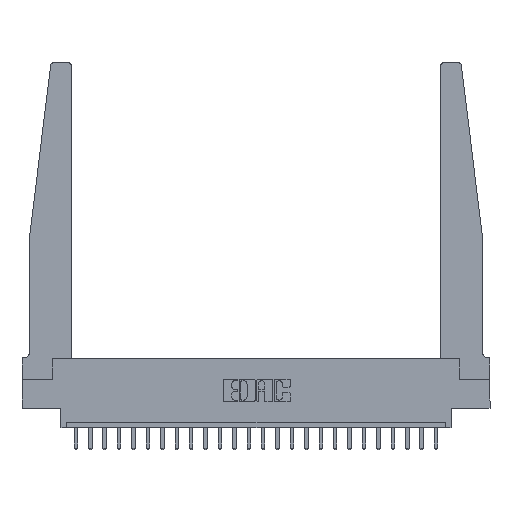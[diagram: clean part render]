
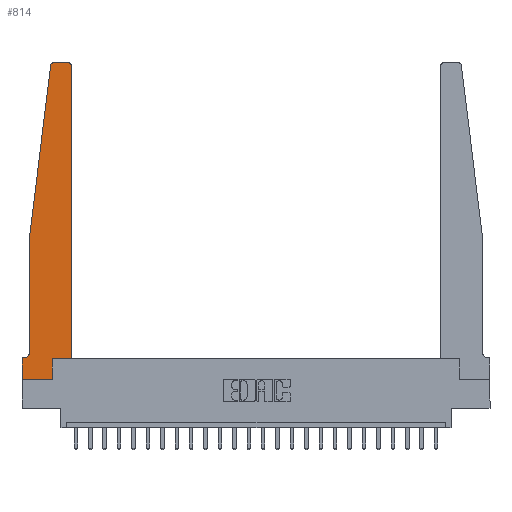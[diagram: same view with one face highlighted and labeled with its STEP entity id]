
A CAD part, top view. The second image highlights one B-rep face of the part: STEP entity #814.
In plain terms, the highlighted planar face has unit normal (0, 0, 1).
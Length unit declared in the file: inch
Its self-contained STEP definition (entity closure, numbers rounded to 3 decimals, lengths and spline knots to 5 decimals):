
#510 = CARTESIAN_POINT ( 'NONE',  ( 0.015, 0.1875, 0.37 ) ) ;
#647 = LINE ( 'NONE', #21854, #4325 ) ;
#814 = ADVANCED_FACE ( 'NONE', ( #14482 ), #22497, .T. ) ;
#943 = VECTOR ( 'NONE', #6972, 39.37008 ) ;
#951 = CARTESIAN_POINT ( 'NONE',  ( 0., 0.1875, 0.37 ) ) ;
#1083 = DIRECTION ( 'NONE',  ( -0.122, -0.992, 0. ) ) ;
#1521 = CARTESIAN_POINT ( 'NONE',  ( 0.065, 0.1875, 0.37 ) ) ;
#2001 = EDGE_CURVE ( 'NONE', #9670, #10453, #11016, .T. ) ;
#2574 = ORIENTED_EDGE ( 'NONE', *, *, #3898, .T. ) ;
#2710 = VECTOR ( 'NONE', #20723, 39.37008 ) ;
#2790 = ORIENTED_EDGE ( 'NONE', *, *, #19519, .T. ) ;
#3064 = ORIENTED_EDGE ( 'NONE', *, *, #8582, .T. ) ;
#3898 = EDGE_CURVE ( 'NONE', #12714, #7843, #4428, .T. ) ;
#3945 = CARTESIAN_POINT ( 'NONE',  ( 0.395, 2.72, 0.37 ) ) ;
#4252 = CARTESIAN_POINT ( 'NONE',  ( 0.395, 2.75, 0.37 ) ) ;
#4325 = VECTOR ( 'NONE', #9304, 39.37008 ) ;
#4428 = LINE ( 'NONE', #17457, #2710 ) ;
#4794 = CARTESIAN_POINT ( 'NONE',  ( 0.425, 0.18, 0.37 ) ) ;
#5068 = DIRECTION ( 'NONE',  ( -1., 0., 0. ) ) ;
#5776 = DIRECTION ( 'NONE',  ( 0., 0., 1. ) ) ;
#5869 = EDGE_LOOP ( 'NONE', ( #23331, #13779, #8024, #22298, #11572, #3064, #17739, #11945, #2790, #2574, #11406, #8471 ) ) ;
#5877 = LINE ( 'NONE', #12318, #21608 ) ;
#6385 = CARTESIAN_POINT ( 'NONE',  ( 0.425, 2.72, 0.37 ) ) ;
#6489 = DIRECTION ( 'NONE',  ( 1., 0., 0. ) ) ;
#6539 = DIRECTION ( 'NONE',  ( -1., 0., 0. ) ) ;
#6719 = CARTESIAN_POINT ( 'NONE',  ( 0.2605, 0.18, 0.37 ) ) ;
#6972 = DIRECTION ( 'NONE',  ( -1., 0., 0. ) ) ;
#7675 = VERTEX_POINT ( 'NONE', #22727 ) ;
#7843 = VERTEX_POINT ( 'NONE', #10070 ) ;
#8024 = ORIENTED_EDGE ( 'NONE', *, *, #13132, .T. ) ;
#8038 = LINE ( 'NONE', #4794, #15122 ) ;
#8423 = EDGE_CURVE ( 'NONE', #10469, #11655, #21215, .T. ) ;
#8471 = ORIENTED_EDGE ( 'NONE', *, *, #2001, .T. ) ;
#8582 = EDGE_CURVE ( 'NONE', #20095, #7675, #20371, .T. ) ;
#9175 = EDGE_CURVE ( 'NONE', #10453, #10469, #10291, .T. ) ;
#9304 = DIRECTION ( 'NONE',  ( 0., -1., 0. ) ) ;
#9467 = AXIS2_PLACEMENT_3D ( 'NONE', #951, #15490, #6489 ) ;
#9670 = VERTEX_POINT ( 'NONE', #6385 ) ;
#10070 = CARTESIAN_POINT ( 'NONE',  ( 0.425, 0.18, 0.37 ) ) ;
#10280 = DIRECTION ( 'NONE',  ( 0., 1., 0. ) ) ;
#10291 = LINE ( 'NONE', #16037, #12256 ) ;
#10453 = VERTEX_POINT ( 'NONE', #4252 ) ;
#10469 = VERTEX_POINT ( 'NONE', #20608 ) ;
#10473 = CARTESIAN_POINT ( 'NONE',  ( 0.065, 1.25, 0.37 ) ) ;
#10687 = DIRECTION ( 'NONE',  ( 1., 0., 0. ) ) ;
#11016 = CIRCLE ( 'NONE', #13734, 0.03 ) ;
#11231 = VECTOR ( 'NONE', #12220, 39.37008 ) ;
#11406 = ORIENTED_EDGE ( 'NONE', *, *, #15987, .T. ) ;
#11572 = ORIENTED_EDGE ( 'NONE', *, *, #11796, .T. ) ;
#11655 = VERTEX_POINT ( 'NONE', #13926 ) ;
#11796 = EDGE_CURVE ( 'NONE', #17698, #20095, #22821, .T. ) ;
#11915 = CARTESIAN_POINT ( 'NONE',  ( 0.015, 0.2375, 0.37 ) ) ;
#11945 = ORIENTED_EDGE ( 'NONE', *, *, #14440, .T. ) ;
#12220 = DIRECTION ( 'NONE',  ( 0., -1., 0. ) ) ;
#12256 = VECTOR ( 'NONE', #5068, 39.37008 ) ;
#12270 = VERTEX_POINT ( 'NONE', #10473 ) ;
#12318 = CARTESIAN_POINT ( 'NONE',  ( 0., 0., 0.37 ) ) ;
#12375 = LINE ( 'NONE', #17498, #11231 ) ;
#12511 = DIRECTION ( 'NONE',  ( 0., 1., 0. ) ) ;
#12714 = VERTEX_POINT ( 'NONE', #21236 ) ;
#13132 = EDGE_CURVE ( 'NONE', #11655, #12270, #19942, .T. ) ;
#13734 = AXIS2_PLACEMENT_3D ( 'NONE', #3945, #5776, #16731 ) ;
#13779 = ORIENTED_EDGE ( 'NONE', *, *, #8423, .T. ) ;
#13926 = CARTESIAN_POINT ( 'NONE',  ( 0.24675, 2.72367, 0.37 ) ) ;
#14440 = EDGE_CURVE ( 'NONE', #17237, #18864, #5877, .T. ) ;
#14482 = FACE_OUTER_BOUND ( 'NONE', #5869, .T. ) ;
#14658 = VECTOR ( 'NONE', #10280, 39.37008 ) ;
#15122 = VECTOR ( 'NONE', #12511, 39.37008 ) ;
#15490 = DIRECTION ( 'NONE',  ( 0., 0., 1. ) ) ;
#15699 = DIRECTION ( 'NONE',  ( 0., 0., -1. ) ) ;
#15796 = VECTOR ( 'NONE', #1083, 39.37008 ) ;
#15987 = EDGE_CURVE ( 'NONE', #7843, #9670, #8038, .T. ) ;
#16037 = CARTESIAN_POINT ( 'NONE',  ( 0.25, 2.75, 0.37 ) ) ;
#16536 = CARTESIAN_POINT ( 'NONE',  ( 0., 0., 0.37 ) ) ;
#16693 = DIRECTION ( 'NONE',  ( 0., 0., 1. ) ) ;
#16731 = DIRECTION ( 'NONE',  ( 1., 0., 0. ) ) ;
#16920 = EDGE_CURVE ( 'NONE', #12270, #17698, #647, .T. ) ;
#17237 = VERTEX_POINT ( 'NONE', #16536 ) ;
#17457 = CARTESIAN_POINT ( 'NONE',  ( 0.425, 0.18, 0.37 ) ) ;
#17498 = CARTESIAN_POINT ( 'NONE',  ( 0., 0., 0.37 ) ) ;
#17694 = LINE ( 'NONE', #6719, #14658 ) ;
#17698 = VERTEX_POINT ( 'NONE', #22851 ) ;
#17739 = ORIENTED_EDGE ( 'NONE', *, *, #19137, .T. ) ;
#18043 = AXIS2_PLACEMENT_3D ( 'NONE', #11915, #15699, #6539 ) ;
#18507 = DIRECTION ( 'NONE',  ( 1., 0., 0. ) ) ;
#18864 = VERTEX_POINT ( 'NONE', #21161 ) ;
#19137 = EDGE_CURVE ( 'NONE', #7675, #17237, #12375, .T. ) ;
#19519 = EDGE_CURVE ( 'NONE', #18864, #12714, #17694, .T. ) ;
#19942 = LINE ( 'NONE', #20598, #15796 ) ;
#20060 = AXIS2_PLACEMENT_3D ( 'NONE', #22211, #16693, #18507 ) ;
#20095 = VERTEX_POINT ( 'NONE', #510 ) ;
#20371 = LINE ( 'NONE', #1521, #943 ) ;
#20598 = CARTESIAN_POINT ( 'NONE',  ( 0.065, 1.25, 0.37 ) ) ;
#20608 = CARTESIAN_POINT ( 'NONE',  ( 0.27653, 2.75, 0.37 ) ) ;
#20723 = DIRECTION ( 'NONE',  ( 1., 0., 0. ) ) ;
#21161 = CARTESIAN_POINT ( 'NONE',  ( 0.2605, 0., 0.37 ) ) ;
#21215 = CIRCLE ( 'NONE', #20060, 0.03 ) ;
#21236 = CARTESIAN_POINT ( 'NONE',  ( 0.2605, 0.18, 0.37 ) ) ;
#21608 = VECTOR ( 'NONE', #10687, 39.37008 ) ;
#21854 = CARTESIAN_POINT ( 'NONE',  ( 0.065, 1.25, 0.37 ) ) ;
#22211 = CARTESIAN_POINT ( 'NONE',  ( 0.27653, 2.72, 0.37 ) ) ;
#22298 = ORIENTED_EDGE ( 'NONE', *, *, #16920, .T. ) ;
#22497 = PLANE ( 'NONE',  #9467 ) ;
#22727 = CARTESIAN_POINT ( 'NONE',  ( 0., 0.1875, 0.37 ) ) ;
#22821 = CIRCLE ( 'NONE', #18043, 0.05 ) ;
#22851 = CARTESIAN_POINT ( 'NONE',  ( 0.065, 0.2375, 0.37 ) ) ;
#23331 = ORIENTED_EDGE ( 'NONE', *, *, #9175, .T. ) ;
